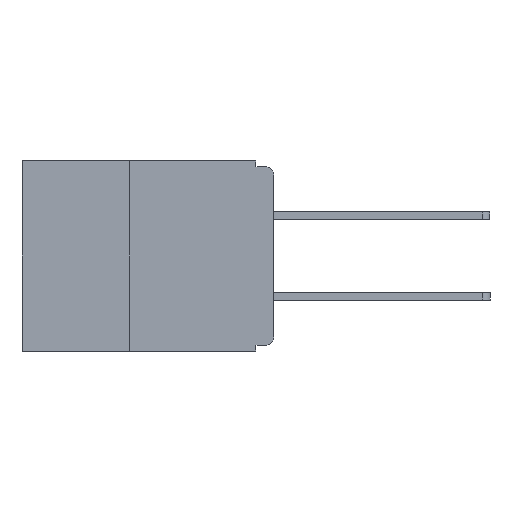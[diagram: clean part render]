
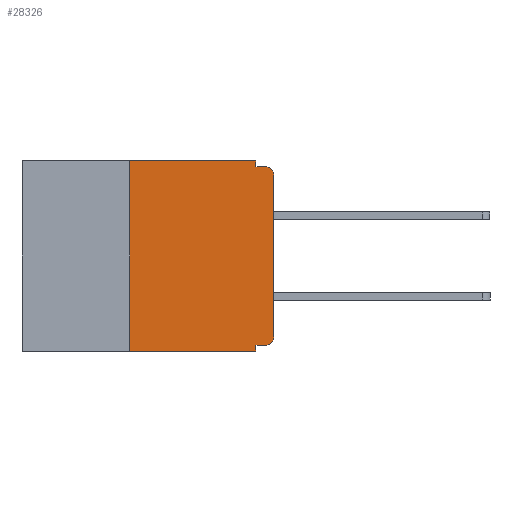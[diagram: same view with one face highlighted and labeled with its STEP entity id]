
A CAD part, left-side view. The second image highlights one B-rep face of the part: STEP entity #28326.
In plain terms, the highlighted planar face has unit normal (-1, 0, 0).
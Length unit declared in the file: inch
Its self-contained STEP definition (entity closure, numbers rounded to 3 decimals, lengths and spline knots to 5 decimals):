
#402 = LINE ( 'NONE', #20764, #2118 ) ;
#1171 = CARTESIAN_POINT ( 'NONE',  ( 0., 0.015, -0.01 ) ) ;
#1173 = CARTESIAN_POINT ( 'NONE',  ( 0., 0.031, 0. ) ) ;
#1543 = LINE ( 'NONE', #17957, #14453 ) ;
#2118 = VECTOR ( 'NONE', #21499, 39.37008 ) ;
#2331 = VERTEX_POINT ( 'NONE', #9820 ) ;
#2460 = CARTESIAN_POINT ( 'NONE',  ( 0., 0.031, -0.32 ) ) ;
#2645 = CIRCLE ( 'NONE', #31079, 0.015 ) ;
#3054 = CARTESIAN_POINT ( 'NONE',  ( 0., 0., -0.025 ) ) ;
#3280 = ORIENTED_EDGE ( 'NONE', *, *, #5119, .T. ) ;
#3337 = CARTESIAN_POINT ( 'NONE',  ( 0., 0.015, -0.025 ) ) ;
#3599 = EDGE_CURVE ( 'NONE', #2331, #19421, #2645, .T. ) ;
#3814 = VERTEX_POINT ( 'NONE', #33311 ) ;
#3939 = DIRECTION ( 'NONE',  ( 0., 0., -1. ) ) ;
#4025 = PLANE ( 'NONE',  #31978 ) ;
#4771 = EDGE_CURVE ( 'NONE', #28715, #14099, #402, .T. ) ;
#4941 = CARTESIAN_POINT ( 'NONE',  ( 0., 0.25, 0. ) ) ;
#5119 = EDGE_CURVE ( 'NONE', #19421, #30048, #31887, .T. ) ;
#6092 = DIRECTION ( 'NONE',  ( 0., 0., -1. ) ) ;
#6787 = DIRECTION ( 'NONE',  ( 1., 0., 0. ) ) ;
#7020 = VERTEX_POINT ( 'NONE', #34547 ) ;
#7202 = ORIENTED_EDGE ( 'NONE', *, *, #28555, .T. ) ;
#7606 = VECTOR ( 'NONE', #18747, 39.37008 ) ;
#8091 = AXIS2_PLACEMENT_3D ( 'NONE', #3337, #22468, #6092 ) ;
#8334 = LINE ( 'NONE', #21991, #22469 ) ;
#9023 = CARTESIAN_POINT ( 'NONE',  ( 0., 0., 0. ) ) ;
#9076 = DIRECTION ( 'NONE',  ( 0., 0., -1. ) ) ;
#9105 = DIRECTION ( 'NONE',  ( 0., 0., 1. ) ) ;
#9706 = DIRECTION ( 'NONE',  ( 0., 1., 0. ) ) ;
#9820 = CARTESIAN_POINT ( 'NONE',  ( 0., 0.015, -0.32 ) ) ;
#10498 = LINE ( 'NONE', #19921, #31261 ) ;
#10565 = LINE ( 'NONE', #1173, #15266 ) ;
#11548 = ORIENTED_EDGE ( 'NONE', *, *, #23740, .F. ) ;
#11954 = ORIENTED_EDGE ( 'NONE', *, *, #29599, .F. ) ;
#13247 = ORIENTED_EDGE ( 'NONE', *, *, #3599, .T. ) ;
#13309 = DIRECTION ( 'NONE',  ( 0., -1., 0. ) ) ;
#13656 = ORIENTED_EDGE ( 'NONE', *, *, #30295, .F. ) ;
#14099 = VERTEX_POINT ( 'NONE', #1171 ) ;
#14359 = EDGE_CURVE ( 'NONE', #24768, #3814, #32091, .T. ) ;
#14438 = VERTEX_POINT ( 'NONE', #2460 ) ;
#14453 = VECTOR ( 'NONE', #9706, 39.37008 ) ;
#14492 = CARTESIAN_POINT ( 'NONE',  ( 0., 0.437, 0. ) ) ;
#14629 = CARTESIAN_POINT ( 'NONE',  ( 0., 0., -0.305 ) ) ;
#15266 = VECTOR ( 'NONE', #3939, 39.37008 ) ;
#16667 = DIRECTION ( 'NONE',  ( 0., 0., 1. ) ) ;
#16700 = CARTESIAN_POINT ( 'NONE',  ( 0., 0.031, -0.01 ) ) ;
#17474 = ORIENTED_EDGE ( 'NONE', *, *, #4771, .F. ) ;
#17816 = CARTESIAN_POINT ( 'NONE',  ( 0., 0.015, -0.305 ) ) ;
#17957 = CARTESIAN_POINT ( 'NONE',  ( 0., 0., -0.32 ) ) ;
#18733 = ORIENTED_EDGE ( 'NONE', *, *, #26793, .T. ) ;
#18747 = DIRECTION ( 'NONE',  ( 0., -1., 0. ) ) ;
#19421 = VERTEX_POINT ( 'NONE', #14629 ) ;
#19855 = DIRECTION ( 'NONE',  ( -1., 0., 0. ) ) ;
#19921 = CARTESIAN_POINT ( 'NONE',  ( 0., 0.031, -0.33 ) ) ;
#20092 = DIRECTION ( 'NONE',  ( 0., 0., -1. ) ) ;
#20764 = CARTESIAN_POINT ( 'NONE',  ( 0., 0., -0.01 ) ) ;
#21389 = CIRCLE ( 'NONE', #8091, 0.015 ) ;
#21499 = DIRECTION ( 'NONE',  ( 0., -1., 0. ) ) ;
#21991 = CARTESIAN_POINT ( 'NONE',  ( 0., 0.25, -0.33 ) ) ;
#22468 = DIRECTION ( 'NONE',  ( -1., 0., 0. ) ) ;
#22469 = VECTOR ( 'NONE', #16667, 39.37008 ) ;
#22562 = ORIENTED_EDGE ( 'NONE', *, *, #31040, .F. ) ;
#23740 = EDGE_CURVE ( 'NONE', #2331, #14438, #1543, .T. ) ;
#24165 = CARTESIAN_POINT ( 'NONE',  ( 0., 0.437, -0.33 ) ) ;
#24749 = VECTOR ( 'NONE', #9105, 39.37008 ) ;
#24768 = VERTEX_POINT ( 'NONE', #4941 ) ;
#25852 = DIRECTION ( 'NONE',  ( 0., 0., -1. ) ) ;
#26793 = EDGE_CURVE ( 'NONE', #30048, #14099, #21389, .T. ) ;
#27221 = ORIENTED_EDGE ( 'NONE', *, *, #14359, .F. ) ;
#27285 = EDGE_LOOP ( 'NONE', ( #3280, #18733, #17474, #11954, #27221, #13656, #7202, #22562, #11548, #13247 ) ) ;
#28326 = ADVANCED_FACE ( 'NONE', ( #31419 ), #4025, .F. ) ;
#28481 = LINE ( 'NONE', #24165, #7606 ) ;
#28555 = EDGE_CURVE ( 'NONE', #34606, #7020, #28481, .T. ) ;
#28715 = VERTEX_POINT ( 'NONE', #16700 ) ;
#29532 = CARTESIAN_POINT ( 'NONE',  ( 0., 0.437, 0. ) ) ;
#29599 = EDGE_CURVE ( 'NONE', #3814, #28715, #10565, .T. ) ;
#30048 = VERTEX_POINT ( 'NONE', #3054 ) ;
#30295 = EDGE_CURVE ( 'NONE', #34606, #24768, #8334, .T. ) ;
#31040 = EDGE_CURVE ( 'NONE', #14438, #7020, #10498, .T. ) ;
#31079 = AXIS2_PLACEMENT_3D ( 'NONE', #17816, #19855, #20092 ) ;
#31261 = VECTOR ( 'NONE', #9076, 39.37008 ) ;
#31419 = FACE_OUTER_BOUND ( 'NONE', #27285, .T. ) ;
#31887 = LINE ( 'NONE', #9023, #24749 ) ;
#31978 = AXIS2_PLACEMENT_3D ( 'NONE', #14492, #6787, #25852 ) ;
#32091 = LINE ( 'NONE', #29532, #32912 ) ;
#32625 = CARTESIAN_POINT ( 'NONE',  ( 0., 0.25, -0.33 ) ) ;
#32912 = VECTOR ( 'NONE', #13309, 39.37008 ) ;
#33311 = CARTESIAN_POINT ( 'NONE',  ( 0., 0.031, 0. ) ) ;
#34547 = CARTESIAN_POINT ( 'NONE',  ( 0., 0.031, -0.33 ) ) ;
#34606 = VERTEX_POINT ( 'NONE', #32625 ) ;
